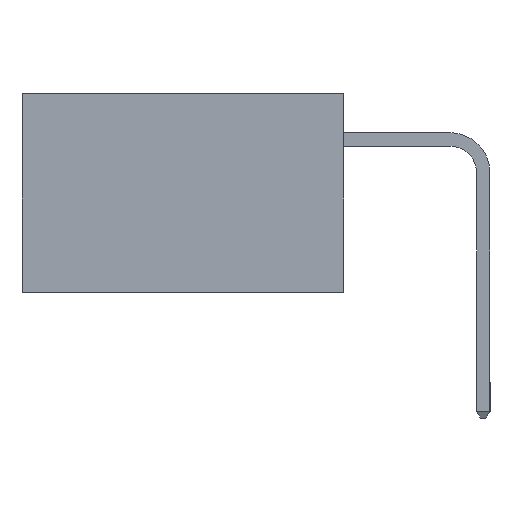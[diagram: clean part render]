
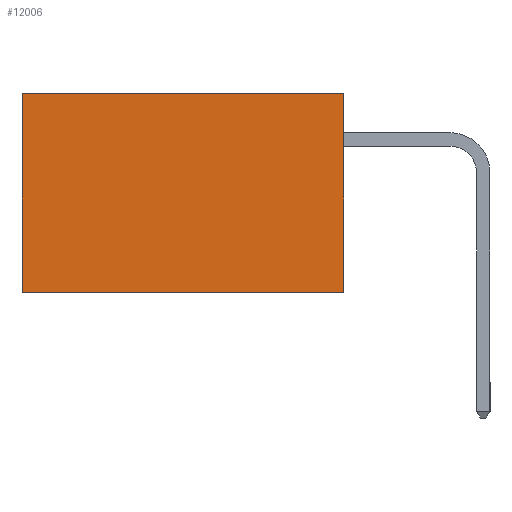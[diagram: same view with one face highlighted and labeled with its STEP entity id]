
A CAD part, left-side view. The second image highlights one B-rep face of the part: STEP entity #12006.
In plain terms, the highlighted planar face has unit normal (-1, 0, 0).
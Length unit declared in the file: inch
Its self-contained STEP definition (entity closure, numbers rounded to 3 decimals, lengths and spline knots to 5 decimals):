
#117 = VECTOR ( 'NONE', #2315, 39.37008 ) ;
#258 = VERTEX_POINT ( 'NONE', #7766 ) ;
#544 = AXIS2_PLACEMENT_3D ( 'NONE', #703, #10489, #4585 ) ;
#689 = DIRECTION ( 'NONE',  ( 0., 0., -1. ) ) ;
#703 = CARTESIAN_POINT ( 'NONE',  ( 0.298, 0., 0. ) ) ;
#741 = LINE ( 'NONE', #11644, #5572 ) ;
#827 = CARTESIAN_POINT ( 'NONE',  ( 0.298, 0.6, -0.37 ) ) ;
#1379 = VERTEX_POINT ( 'NONE', #4133 ) ;
#1389 = FACE_OUTER_BOUND ( 'NONE', #8543, .T. ) ;
#1942 = ORIENTED_EDGE ( 'NONE', *, *, #5871, .T. ) ;
#2016 = VECTOR ( 'NONE', #689, 39.37008 ) ;
#2315 = DIRECTION ( 'NONE',  ( 0., 0., -1. ) ) ;
#2365 = LINE ( 'NONE', #8166, #117 ) ;
#2709 = VERTEX_POINT ( 'NONE', #827 ) ;
#4103 = LINE ( 'NONE', #5303, #6385 ) ;
#4133 = CARTESIAN_POINT ( 'NONE',  ( 0.298, 0., 0. ) ) ;
#4550 = PLANE ( 'NONE',  #544 ) ;
#4585 = DIRECTION ( 'NONE',  ( 0., 0., -1. ) ) ;
#5303 = CARTESIAN_POINT ( 'NONE',  ( 0.298, 0., -0.37 ) ) ;
#5379 = VERTEX_POINT ( 'NONE', #10864 ) ;
#5572 = VECTOR ( 'NONE', #11424, 39.37008 ) ;
#5871 = EDGE_CURVE ( 'NONE', #1379, #258, #741, .T. ) ;
#6385 = VECTOR ( 'NONE', #12173, 39.37008 ) ;
#7766 = CARTESIAN_POINT ( 'NONE',  ( 0.298, 0.6, 0. ) ) ;
#8166 = CARTESIAN_POINT ( 'NONE',  ( 0.298, 0., 0. ) ) ;
#8473 = CARTESIAN_POINT ( 'NONE',  ( 0.298, 0.6, 0. ) ) ;
#8543 = EDGE_LOOP ( 'NONE', ( #10806, #11361, #10928, #1942 ) ) ;
#8934 = EDGE_CURVE ( 'NONE', #1379, #5379, #2365, .T. ) ;
#9813 = LINE ( 'NONE', #8473, #2016 ) ;
#10489 = DIRECTION ( 'NONE',  ( 1., 0., 0. ) ) ;
#10718 = EDGE_CURVE ( 'NONE', #258, #2709, #9813, .T. ) ;
#10806 = ORIENTED_EDGE ( 'NONE', *, *, #10718, .T. ) ;
#10864 = CARTESIAN_POINT ( 'NONE',  ( 0.298, 0., -0.37 ) ) ;
#10928 = ORIENTED_EDGE ( 'NONE', *, *, #8934, .F. ) ;
#11361 = ORIENTED_EDGE ( 'NONE', *, *, #11861, .F. ) ;
#11424 = DIRECTION ( 'NONE',  ( 0., 1., 0. ) ) ;
#11644 = CARTESIAN_POINT ( 'NONE',  ( 0.298, 0., 0. ) ) ;
#11861 = EDGE_CURVE ( 'NONE', #5379, #2709, #4103, .T. ) ;
#12006 = ADVANCED_FACE ( 'NONE', ( #1389 ), #4550, .F. ) ;
#12173 = DIRECTION ( 'NONE',  ( 0., 1., 0. ) ) ;
